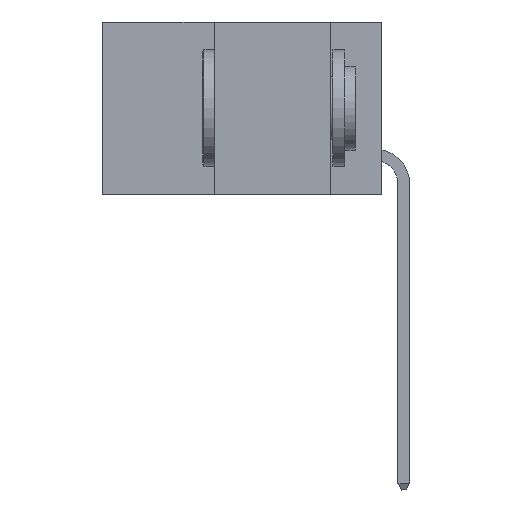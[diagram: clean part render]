
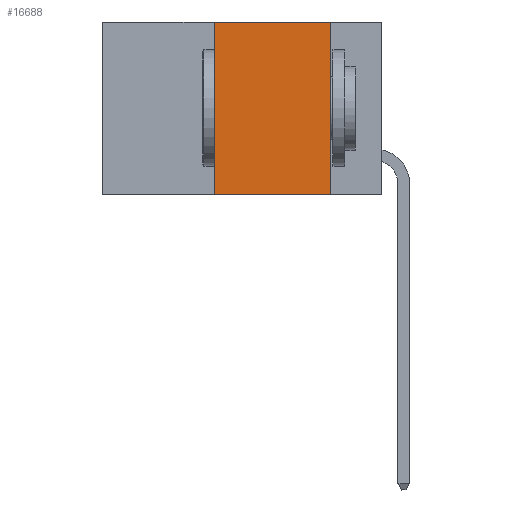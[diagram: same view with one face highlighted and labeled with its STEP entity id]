
A CAD part, left-side view. The second image highlights one B-rep face of the part: STEP entity #16688.
In plain terms, the highlighted planar face has unit normal (-1, 0, 0).
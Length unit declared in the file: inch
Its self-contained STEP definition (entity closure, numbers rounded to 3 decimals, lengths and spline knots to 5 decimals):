
#2758 = EDGE_CURVE ( 'NONE', #5912, #25959, #20121, .T. ) ;
#3241 = ORIENTED_EDGE ( 'NONE', *, *, #2758, .F. ) ;
#3562 = CARTESIAN_POINT ( 'NONE',  ( 0., 0.6, 0. ) ) ;
#3635 = CARTESIAN_POINT ( 'NONE',  ( 0., 0.6, 0. ) ) ;
#3714 = LINE ( 'NONE', #3635, #21019 ) ;
#3775 = DIRECTION ( 'NONE',  ( 0., 0., -1. ) ) ;
#3779 = EDGE_CURVE ( 'NONE', #18446, #14642, #7512, .T. ) ;
#4758 = ORIENTED_EDGE ( 'NONE', *, *, #20375, .T. ) ;
#5912 = VERTEX_POINT ( 'NONE', #9181 ) ;
#6726 = CARTESIAN_POINT ( 'NONE',  ( 0., 0.6, -0.37 ) ) ;
#7512 = LINE ( 'NONE', #7948, #16696 ) ;
#7948 = CARTESIAN_POINT ( 'NONE',  ( 0., 0.36, 0. ) ) ;
#9181 = CARTESIAN_POINT ( 'NONE',  ( 0., 0.11, 0. ) ) ;
#9296 = DIRECTION ( 'NONE',  ( 0., 0., 1. ) ) ;
#10938 = FACE_OUTER_BOUND ( 'NONE', #17412, .T. ) ;
#11361 = DIRECTION ( 'NONE',  ( 0., -1., 0. ) ) ;
#12738 = LINE ( 'NONE', #6726, #18834 ) ;
#14182 = CARTESIAN_POINT ( 'NONE',  ( 0., 0.36, 0. ) ) ;
#14642 = VERTEX_POINT ( 'NONE', #14182 ) ;
#16688 = ADVANCED_FACE ( 'NONE', ( #10938 ), #18389, .F. ) ;
#16696 = VECTOR ( 'NONE', #9296, 39.37008 ) ;
#16746 = DIRECTION ( 'NONE',  ( 0., -1., 0. ) ) ;
#16999 = CARTESIAN_POINT ( 'NONE',  ( 0., 0.11, 0. ) ) ;
#17412 = EDGE_LOOP ( 'NONE', ( #3241, #19523, #25246, #4758 ) ) ;
#18389 = PLANE ( 'NONE',  #26735 ) ;
#18446 = VERTEX_POINT ( 'NONE', #25953 ) ;
#18834 = VECTOR ( 'NONE', #11361, 39.37008 ) ;
#19523 = ORIENTED_EDGE ( 'NONE', *, *, #27360, .F. ) ;
#20121 = LINE ( 'NONE', #16999, #22497 ) ;
#20375 = EDGE_CURVE ( 'NONE', #18446, #25959, #12738, .T. ) ;
#20593 = CARTESIAN_POINT ( 'NONE',  ( 0., 0.11, -0.37 ) ) ;
#20654 = DIRECTION ( 'NONE',  ( 0., 0., -1. ) ) ;
#20830 = DIRECTION ( 'NONE',  ( 1., 0., 0. ) ) ;
#21019 = VECTOR ( 'NONE', #16746, 39.37008 ) ;
#22497 = VECTOR ( 'NONE', #3775, 39.37008 ) ;
#25246 = ORIENTED_EDGE ( 'NONE', *, *, #3779, .F. ) ;
#25953 = CARTESIAN_POINT ( 'NONE',  ( 0., 0.36, -0.37 ) ) ;
#25959 = VERTEX_POINT ( 'NONE', #20593 ) ;
#26735 = AXIS2_PLACEMENT_3D ( 'NONE', #3562, #20830, #20654 ) ;
#27360 = EDGE_CURVE ( 'NONE', #14642, #5912, #3714, .T. ) ;
